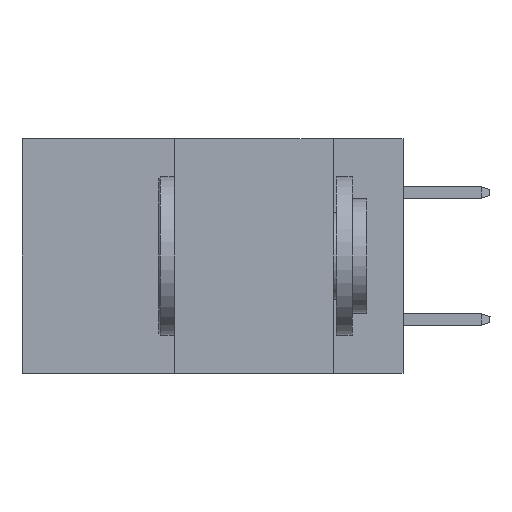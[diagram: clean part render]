
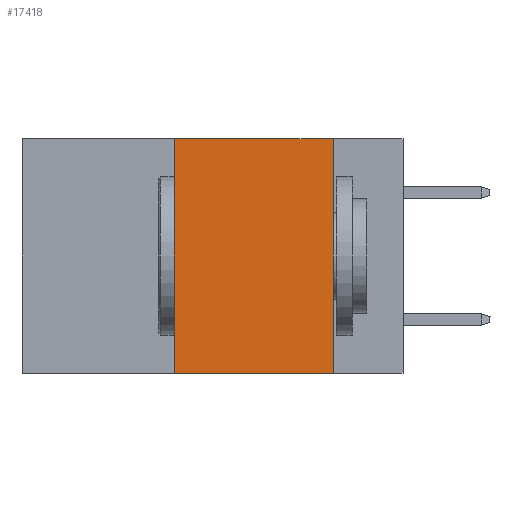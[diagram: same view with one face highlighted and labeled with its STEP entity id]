
A CAD part, left-side view. The second image highlights one B-rep face of the part: STEP entity #17418.
In plain terms, the highlighted planar face has unit normal (-1, 0, 0).
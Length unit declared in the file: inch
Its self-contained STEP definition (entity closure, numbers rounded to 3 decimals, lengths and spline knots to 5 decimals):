
#143 = CARTESIAN_POINT ( 'NONE',  ( 0., 0.36, 0. ) ) ;
#334 = VERTEX_POINT ( 'NONE', #15689 ) ;
#403 = DIRECTION ( 'NONE',  ( 0., -1., 0. ) ) ;
#666 = VECTOR ( 'NONE', #1764, 39.37008 ) ;
#766 = LINE ( 'NONE', #15829, #3904 ) ;
#1010 = EDGE_LOOP ( 'NONE', ( #2880, #4425, #17495, #6684 ) ) ;
#1117 = LINE ( 'NONE', #13319, #4635 ) ;
#1424 = CARTESIAN_POINT ( 'NONE',  ( 0., 0.11, 0. ) ) ;
#1764 = DIRECTION ( 'NONE',  ( 0., 0., 1. ) ) ;
#2880 = ORIENTED_EDGE ( 'NONE', *, *, #13823, .F. ) ;
#3072 = VERTEX_POINT ( 'NONE', #1424 ) ;
#3904 = VECTOR ( 'NONE', #11811, 39.37008 ) ;
#4425 = ORIENTED_EDGE ( 'NONE', *, *, #4620, .F. ) ;
#4620 = EDGE_CURVE ( 'NONE', #334, #3072, #1117, .T. ) ;
#4635 = VECTOR ( 'NONE', #10340, 39.37008 ) ;
#5346 = PLANE ( 'NONE',  #17538 ) ;
#5954 = VERTEX_POINT ( 'NONE', #14150 ) ;
#6684 = ORIENTED_EDGE ( 'NONE', *, *, #10797, .T. ) ;
#6923 = CARTESIAN_POINT ( 'NONE',  ( 0., 0.6, 0. ) ) ;
#7715 = LINE ( 'NONE', #143, #666 ) ;
#9593 = VERTEX_POINT ( 'NONE', #17940 ) ;
#10340 = DIRECTION ( 'NONE',  ( 0., -1., 0. ) ) ;
#10551 = EDGE_CURVE ( 'NONE', #5954, #334, #7715, .T. ) ;
#10797 = EDGE_CURVE ( 'NONE', #5954, #9593, #12069, .T. ) ;
#11099 = DIRECTION ( 'NONE',  ( 0., 0., -1. ) ) ;
#11284 = DIRECTION ( 'NONE',  ( 1., 0., 0. ) ) ;
#11811 = DIRECTION ( 'NONE',  ( 0., 0., -1. ) ) ;
#12069 = LINE ( 'NONE', #15470, #18941 ) ;
#13319 = CARTESIAN_POINT ( 'NONE',  ( 0., 0.6, 0. ) ) ;
#13823 = EDGE_CURVE ( 'NONE', #3072, #9593, #766, .T. ) ;
#14150 = CARTESIAN_POINT ( 'NONE',  ( 0., 0.36, -0.37 ) ) ;
#15470 = CARTESIAN_POINT ( 'NONE',  ( 0., 0.6, -0.37 ) ) ;
#15626 = FACE_OUTER_BOUND ( 'NONE', #1010, .T. ) ;
#15689 = CARTESIAN_POINT ( 'NONE',  ( 0., 0.36, 0. ) ) ;
#15829 = CARTESIAN_POINT ( 'NONE',  ( 0., 0.11, 0. ) ) ;
#17418 = ADVANCED_FACE ( 'NONE', ( #15626 ), #5346, .F. ) ;
#17495 = ORIENTED_EDGE ( 'NONE', *, *, #10551, .F. ) ;
#17538 = AXIS2_PLACEMENT_3D ( 'NONE', #6923, #11284, #11099 ) ;
#17940 = CARTESIAN_POINT ( 'NONE',  ( 0., 0.11, -0.37 ) ) ;
#18941 = VECTOR ( 'NONE', #403, 39.37008 ) ;
